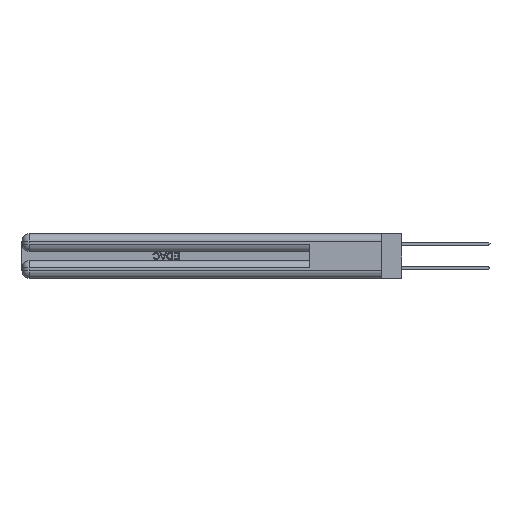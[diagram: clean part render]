
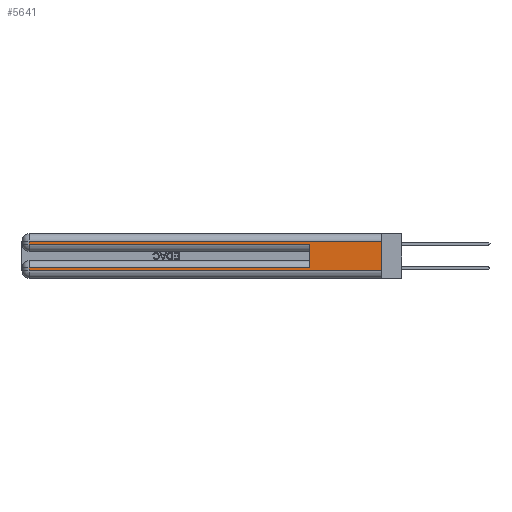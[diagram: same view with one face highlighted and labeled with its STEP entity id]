
A CAD part, left-side view. The second image highlights one B-rep face of the part: STEP entity #5641.
In plain terms, the highlighted planar face has unit normal (-1, 0, 0).
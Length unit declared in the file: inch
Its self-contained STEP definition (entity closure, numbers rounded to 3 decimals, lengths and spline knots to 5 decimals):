
#653 = VECTOR ( 'NONE', #36046, 39.37008 ) ;
#1002 = LINE ( 'NONE', #23021, #19115 ) ;
#1516 = VERTEX_POINT ( 'NONE', #34768 ) ;
#3279 = PLANE ( 'NONE',  #9953 ) ;
#3612 = VERTEX_POINT ( 'NONE', #33895 ) ;
#3765 = VECTOR ( 'NONE', #18608, 39.37008 ) ;
#4549 = CARTESIAN_POINT ( 'NONE',  ( 0., 0., 0.06 ) ) ;
#4592 = VERTEX_POINT ( 'NONE', #17083 ) ;
#4643 = VECTOR ( 'NONE', #30614, 39.37008 ) ;
#5641 = ADVANCED_FACE ( 'NONE', ( #39864 ), #3279, .F. ) ;
#5696 = CARTESIAN_POINT ( 'NONE',  ( 0., 0., 0.06 ) ) ;
#6406 = CARTESIAN_POINT ( 'NONE',  ( 0., 0.6, 0.285 ) ) ;
#8375 = LINE ( 'NONE', #35751, #33558 ) ;
#8580 = EDGE_CURVE ( 'NONE', #1516, #15119, #25072, .T. ) ;
#9155 = ORIENTED_EDGE ( 'NONE', *, *, #33635, .T. ) ;
#9619 = CARTESIAN_POINT ( 'NONE',  ( 0., 0., 0.37 ) ) ;
#9953 = AXIS2_PLACEMENT_3D ( 'NONE', #9619, #27164, #17813 ) ;
#10088 = ORIENTED_EDGE ( 'NONE', *, *, #15771, .F. ) ;
#10438 = DIRECTION ( 'NONE',  ( 0., -1., 0. ) ) ;
#11642 = EDGE_CURVE ( 'NONE', #1516, #24683, #41861, .T. ) ;
#12356 = LINE ( 'NONE', #16897, #4643 ) ;
#12746 = EDGE_CURVE ( 'NONE', #4592, #30239, #8375, .T. ) ;
#13653 = VECTOR ( 'NONE', #34434, 39.37008 ) ;
#14506 = VERTEX_POINT ( 'NONE', #18868 ) ;
#15109 = CARTESIAN_POINT ( 'NONE',  ( 0., 0., 0.085 ) ) ;
#15119 = VERTEX_POINT ( 'NONE', #18218 ) ;
#15771 = EDGE_CURVE ( 'NONE', #4592, #28617, #1002, .T. ) ;
#15999 = EDGE_LOOP ( 'NONE', ( #10088, #33156, #9155, #16347, #27783, #28095, #28270, #33149 ) ) ;
#16347 = ORIENTED_EDGE ( 'NONE', *, *, #23466, .T. ) ;
#16897 = CARTESIAN_POINT ( 'NONE',  ( 0., 2.94, 0.37 ) ) ;
#17083 = CARTESIAN_POINT ( 'NONE',  ( 0., 0., 0.31 ) ) ;
#17813 = DIRECTION ( 'NONE',  ( 0., 0., -1. ) ) ;
#18218 = CARTESIAN_POINT ( 'NONE',  ( 0., 2.94, 0.085 ) ) ;
#18608 = DIRECTION ( 'NONE',  ( 0., 1., 0. ) ) ;
#18868 = CARTESIAN_POINT ( 'NONE',  ( 0., 2.94, 0.06 ) ) ;
#19115 = VECTOR ( 'NONE', #43364, 39.37008 ) ;
#19554 = VECTOR ( 'NONE', #10438, 39.37008 ) ;
#21316 = CARTESIAN_POINT ( 'NONE',  ( 0., 0., 0.285 ) ) ;
#22480 = EDGE_CURVE ( 'NONE', #15119, #14506, #35978, .T. ) ;
#23021 = CARTESIAN_POINT ( 'NONE',  ( 0., 0., 0.37 ) ) ;
#23466 = EDGE_CURVE ( 'NONE', #3612, #24683, #37558, .T. ) ;
#24050 = CARTESIAN_POINT ( 'NONE',  ( 0., 2.94, 0.37 ) ) ;
#24683 = VERTEX_POINT ( 'NONE', #6406 ) ;
#25072 = LINE ( 'NONE', #15109, #3765 ) ;
#27164 = DIRECTION ( 'NONE',  ( 1., 0., 0. ) ) ;
#27783 = ORIENTED_EDGE ( 'NONE', *, *, #11642, .F. ) ;
#28095 = ORIENTED_EDGE ( 'NONE', *, *, #8580, .T. ) ;
#28270 = ORIENTED_EDGE ( 'NONE', *, *, #22480, .T. ) ;
#28617 = VERTEX_POINT ( 'NONE', #5696 ) ;
#30239 = VERTEX_POINT ( 'NONE', #44531 ) ;
#30614 = DIRECTION ( 'NONE',  ( 0., 0., -1. ) ) ;
#32539 = DIRECTION ( 'NONE',  ( 0., 1., 0. ) ) ;
#33149 = ORIENTED_EDGE ( 'NONE', *, *, #42737, .T. ) ;
#33156 = ORIENTED_EDGE ( 'NONE', *, *, #12746, .T. ) ;
#33558 = VECTOR ( 'NONE', #32539, 39.37008 ) ;
#33635 = EDGE_CURVE ( 'NONE', #30239, #3612, #12356, .T. ) ;
#33895 = CARTESIAN_POINT ( 'NONE',  ( 0., 2.94, 0.285 ) ) ;
#34434 = DIRECTION ( 'NONE',  ( 0., 0., -1. ) ) ;
#34768 = CARTESIAN_POINT ( 'NONE',  ( 0., 0.6, 0.085 ) ) ;
#35751 = CARTESIAN_POINT ( 'NONE',  ( 0., 0., 0.31 ) ) ;
#35978 = LINE ( 'NONE', #24050, #13653 ) ;
#36046 = DIRECTION ( 'NONE',  ( 0., -1., 0. ) ) ;
#37558 = LINE ( 'NONE', #21316, #19554 ) ;
#38026 = VECTOR ( 'NONE', #45116, 39.37008 ) ;
#39864 = FACE_OUTER_BOUND ( 'NONE', #15999, .T. ) ;
#41404 = CARTESIAN_POINT ( 'NONE',  ( 0., 0.6, 0.145 ) ) ;
#41861 = LINE ( 'NONE', #41404, #38026 ) ;
#42737 = EDGE_CURVE ( 'NONE', #14506, #28617, #43976, .T. ) ;
#43364 = DIRECTION ( 'NONE',  ( 0., 0., -1. ) ) ;
#43976 = LINE ( 'NONE', #4549, #653 ) ;
#44531 = CARTESIAN_POINT ( 'NONE',  ( 0., 2.94, 0.31 ) ) ;
#45116 = DIRECTION ( 'NONE',  ( 0., 0., 1. ) ) ;
